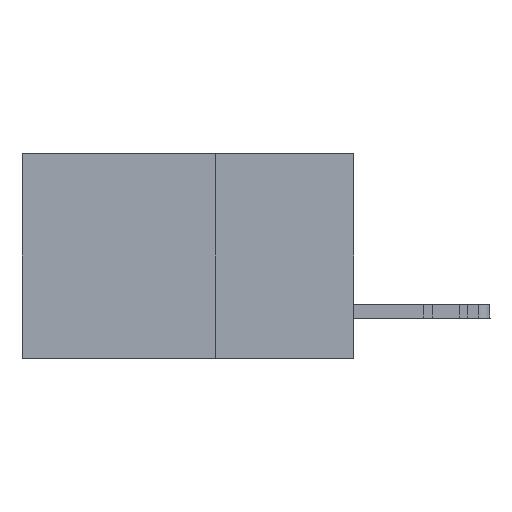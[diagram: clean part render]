
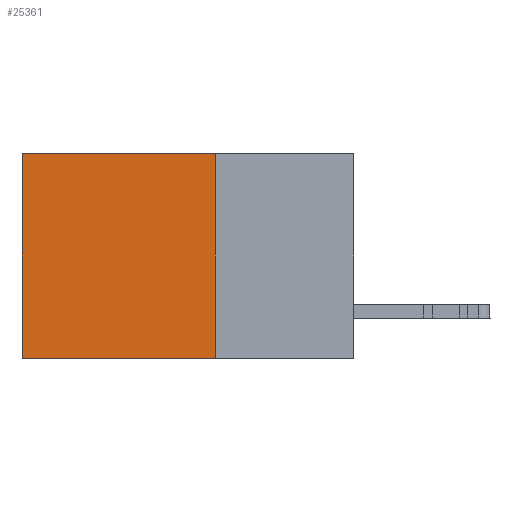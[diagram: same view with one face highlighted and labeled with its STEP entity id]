
A CAD part, left-side view. The second image highlights one B-rep face of the part: STEP entity #25361.
In plain terms, the highlighted planar face has unit normal (-1, 0, 0).
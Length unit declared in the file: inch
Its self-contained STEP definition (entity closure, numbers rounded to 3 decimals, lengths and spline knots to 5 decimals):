
#2883 = AXIS2_PLACEMENT_3D ( 'NONE', #13476, #20579, #29522 ) ;
#2946 = VECTOR ( 'NONE', #22059, 39.37008 ) ;
#3545 = CARTESIAN_POINT ( 'NONE',  ( 0.2875, 0.6, 0. ) ) ;
#4742 = PLANE ( 'NONE',  #2883 ) ;
#6200 = ORIENTED_EDGE ( 'NONE', *, *, #13331, .F. ) ;
#7131 = VERTEX_POINT ( 'NONE', #25972 ) ;
#9350 = EDGE_LOOP ( 'NONE', ( #14513, #32173, #6200, #36797 ) ) ;
#9654 = CARTESIAN_POINT ( 'NONE',  ( 0.2875, 0.6, 0. ) ) ;
#9846 = LINE ( 'NONE', #9654, #2946 ) ;
#11595 = DIRECTION ( 'NONE',  ( 0., 0., -1. ) ) ;
#11773 = VERTEX_POINT ( 'NONE', #20508 ) ;
#13331 = EDGE_CURVE ( 'NONE', #7131, #14482, #27240, .T. ) ;
#13476 = CARTESIAN_POINT ( 'NONE',  ( 0.2875, 0.25, 0. ) ) ;
#13669 = FACE_OUTER_BOUND ( 'NONE', #9350, .T. ) ;
#14424 = VECTOR ( 'NONE', #11595, 39.37008 ) ;
#14482 = VERTEX_POINT ( 'NONE', #30107 ) ;
#14513 = ORIENTED_EDGE ( 'NONE', *, *, #16781, .T. ) ;
#15185 = CARTESIAN_POINT ( 'NONE',  ( 0.2875, 0.25, 0. ) ) ;
#16093 = VECTOR ( 'NONE', #21282, 39.37008 ) ;
#16781 = EDGE_CURVE ( 'NONE', #25263, #11773, #9846, .T. ) ;
#19341 = EDGE_CURVE ( 'NONE', #7131, #25263, #36742, .T. ) ;
#20508 = CARTESIAN_POINT ( 'NONE',  ( 0.2875, 0.6, -0.37 ) ) ;
#20579 = DIRECTION ( 'NONE',  ( 1., 0., 0. ) ) ;
#21282 = DIRECTION ( 'NONE',  ( 0., 1., 0. ) ) ;
#22059 = DIRECTION ( 'NONE',  ( 0., 0., -1. ) ) ;
#24188 = CARTESIAN_POINT ( 'NONE',  ( 0.2875, 0.25, 0. ) ) ;
#25263 = VERTEX_POINT ( 'NONE', #3545 ) ;
#25361 = ADVANCED_FACE ( 'NONE', ( #13669 ), #4742, .F. ) ;
#25866 = VECTOR ( 'NONE', #34114, 39.37008 ) ;
#25972 = CARTESIAN_POINT ( 'NONE',  ( 0.2875, 0.25, 0. ) ) ;
#27240 = LINE ( 'NONE', #24188, #14424 ) ;
#29522 = DIRECTION ( 'NONE',  ( 0., 0., -1. ) ) ;
#30107 = CARTESIAN_POINT ( 'NONE',  ( 0.2875, 0.25, -0.37 ) ) ;
#31071 = CARTESIAN_POINT ( 'NONE',  ( 0.2875, 0.25, -0.37 ) ) ;
#31474 = LINE ( 'NONE', #31071, #25866 ) ;
#32173 = ORIENTED_EDGE ( 'NONE', *, *, #32928, .F. ) ;
#32928 = EDGE_CURVE ( 'NONE', #14482, #11773, #31474, .T. ) ;
#34114 = DIRECTION ( 'NONE',  ( 0., 1., 0. ) ) ;
#36742 = LINE ( 'NONE', #15185, #16093 ) ;
#36797 = ORIENTED_EDGE ( 'NONE', *, *, #19341, .T. ) ;
